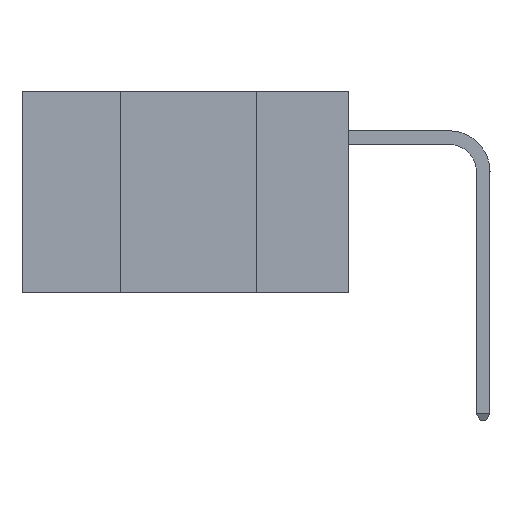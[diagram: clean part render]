
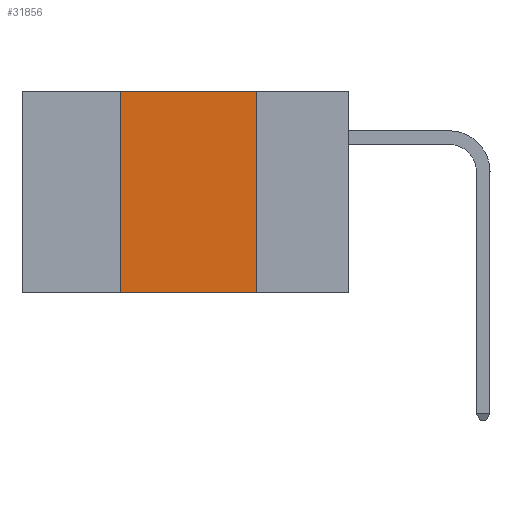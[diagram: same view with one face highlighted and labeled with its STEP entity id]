
A CAD part, left-side view. The second image highlights one B-rep face of the part: STEP entity #31856.
In plain terms, the highlighted planar face has unit normal (-1, 0, 0).
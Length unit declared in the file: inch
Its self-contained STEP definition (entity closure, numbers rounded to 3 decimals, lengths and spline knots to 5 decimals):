
#503 = ORIENTED_EDGE ( 'NONE', *, *, #34199, .F. ) ;
#1509 = DIRECTION ( 'NONE',  ( 0., -1., 0. ) ) ;
#1544 = VERTEX_POINT ( 'NONE', #33948 ) ;
#3968 = FACE_OUTER_BOUND ( 'NONE', #27096, .T. ) ;
#4770 = EDGE_CURVE ( 'NONE', #29306, #26471, #12330, .T. ) ;
#9919 = ORIENTED_EDGE ( 'NONE', *, *, #4770, .T. ) ;
#10339 = LINE ( 'NONE', #26592, #26602 ) ;
#11475 = DIRECTION ( 'NONE',  ( 1., 0., 0. ) ) ;
#12330 = LINE ( 'NONE', #17966, #19938 ) ;
#16459 = ORIENTED_EDGE ( 'NONE', *, *, #36996, .F. ) ;
#17826 = LINE ( 'NONE', #39919, #35034 ) ;
#17966 = CARTESIAN_POINT ( 'NONE',  ( 0., 0.6, -0.37 ) ) ;
#18063 = CARTESIAN_POINT ( 'NONE',  ( 0., 0.42, 0. ) ) ;
#18194 = VECTOR ( 'NONE', #37327, 39.37008 ) ;
#19938 = VECTOR ( 'NONE', #1509, 39.37008 ) ;
#20497 = DIRECTION ( 'NONE',  ( 0., -1., 0. ) ) ;
#21110 = PLANE ( 'NONE',  #28811 ) ;
#25195 = CARTESIAN_POINT ( 'NONE',  ( 0., 0.17, -0.37 ) ) ;
#26471 = VERTEX_POINT ( 'NONE', #25195 ) ;
#26592 = CARTESIAN_POINT ( 'NONE',  ( 0., 0.17, 0. ) ) ;
#26602 = VECTOR ( 'NONE', #29845, 39.37008 ) ;
#27096 = EDGE_LOOP ( 'NONE', ( #16459, #28689, #503, #9919 ) ) ;
#27158 = CARTESIAN_POINT ( 'NONE',  ( 0., 0.42, -0.37 ) ) ;
#27463 = VERTEX_POINT ( 'NONE', #36423 ) ;
#27681 = CARTESIAN_POINT ( 'NONE',  ( 0., 0.6, 0. ) ) ;
#28689 = ORIENTED_EDGE ( 'NONE', *, *, #32103, .F. ) ;
#28811 = AXIS2_PLACEMENT_3D ( 'NONE', #27681, #11475, #34140 ) ;
#29306 = VERTEX_POINT ( 'NONE', #27158 ) ;
#29845 = DIRECTION ( 'NONE',  ( 0., 0., -1. ) ) ;
#31856 = ADVANCED_FACE ( 'NONE', ( #3968 ), #21110, .F. ) ;
#32103 = EDGE_CURVE ( 'NONE', #1544, #27463, #17826, .T. ) ;
#33948 = CARTESIAN_POINT ( 'NONE',  ( 0., 0.42, 0. ) ) ;
#34140 = DIRECTION ( 'NONE',  ( 0., 0., -1. ) ) ;
#34199 = EDGE_CURVE ( 'NONE', #29306, #1544, #35415, .T. ) ;
#35034 = VECTOR ( 'NONE', #20497, 39.37008 ) ;
#35415 = LINE ( 'NONE', #18063, #18194 ) ;
#36423 = CARTESIAN_POINT ( 'NONE',  ( 0., 0.17, 0. ) ) ;
#36996 = EDGE_CURVE ( 'NONE', #27463, #26471, #10339, .T. ) ;
#37327 = DIRECTION ( 'NONE',  ( 0., 0., 1. ) ) ;
#39919 = CARTESIAN_POINT ( 'NONE',  ( 0., 0.6, 0. ) ) ;
